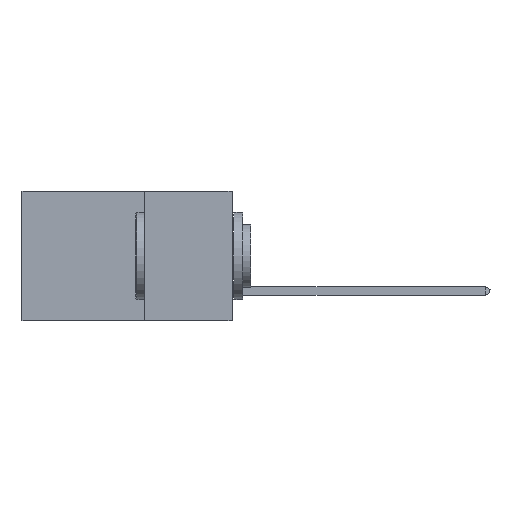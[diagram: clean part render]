
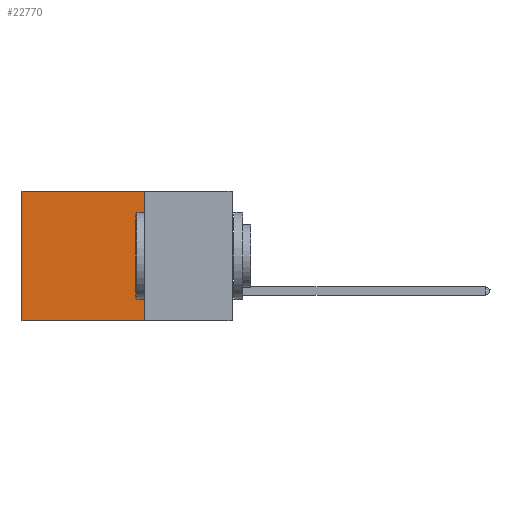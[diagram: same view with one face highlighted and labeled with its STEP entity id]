
A CAD part, left-side view. The second image highlights one B-rep face of the part: STEP entity #22770.
In plain terms, the highlighted planar face has unit normal (-1, 0, 0).
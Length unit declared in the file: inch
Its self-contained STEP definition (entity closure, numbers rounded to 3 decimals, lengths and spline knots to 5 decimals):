
#1149 = PLANE ( 'NONE',  #8282 ) ;
#1723 = VECTOR ( 'NONE', #18892, 39.37008 ) ;
#2273 = VERTEX_POINT ( 'NONE', #7910 ) ;
#2519 = VERTEX_POINT ( 'NONE', #12823 ) ;
#2667 = LINE ( 'NONE', #14567, #1723 ) ;
#3457 = DIRECTION ( 'NONE',  ( 0., 0., -1. ) ) ;
#4595 = VERTEX_POINT ( 'NONE', #13557 ) ;
#5178 = DIRECTION ( 'NONE',  ( 1., 0., 0. ) ) ;
#5205 = ORIENTED_EDGE ( 'NONE', *, *, #19442, .F. ) ;
#5664 = EDGE_CURVE ( 'NONE', #4595, #2273, #2667, .T. ) ;
#6029 = DIRECTION ( 'NONE',  ( 0., 1., 0. ) ) ;
#6645 = CARTESIAN_POINT ( 'NONE',  ( 0.2875, 0.25, 0. ) ) ;
#7910 = CARTESIAN_POINT ( 'NONE',  ( 0.2875, 0.6, -0.37 ) ) ;
#8103 = EDGE_LOOP ( 'NONE', ( #13638, #22200, #5205, #21917 ) ) ;
#8282 = AXIS2_PLACEMENT_3D ( 'NONE', #13088, #5178, #24954 ) ;
#10345 = DIRECTION ( 'NONE',  ( 0., 0., -1. ) ) ;
#10541 = LINE ( 'NONE', #13989, #14677 ) ;
#10616 = LINE ( 'NONE', #18579, #12195 ) ;
#11887 = EDGE_CURVE ( 'NONE', #2519, #2273, #10616, .T. ) ;
#12195 = VECTOR ( 'NONE', #10345, 39.37008 ) ;
#12823 = CARTESIAN_POINT ( 'NONE',  ( 0.2875, 0.6, 0. ) ) ;
#13088 = CARTESIAN_POINT ( 'NONE',  ( 0.2875, 0.25, 0. ) ) ;
#13557 = CARTESIAN_POINT ( 'NONE',  ( 0.2875, 0.25, -0.37 ) ) ;
#13638 = ORIENTED_EDGE ( 'NONE', *, *, #11887, .T. ) ;
#13989 = CARTESIAN_POINT ( 'NONE',  ( 0.2875, 0.25, 0. ) ) ;
#14567 = CARTESIAN_POINT ( 'NONE',  ( 0.2875, 0.25, -0.37 ) ) ;
#14677 = VECTOR ( 'NONE', #6029, 39.37008 ) ;
#15118 = FACE_OUTER_BOUND ( 'NONE', #8103, .T. ) ;
#16511 = CARTESIAN_POINT ( 'NONE',  ( 0.2875, 0.25, 0. ) ) ;
#18579 = CARTESIAN_POINT ( 'NONE',  ( 0.2875, 0.6, 0. ) ) ;
#18892 = DIRECTION ( 'NONE',  ( 0., 1., 0. ) ) ;
#19442 = EDGE_CURVE ( 'NONE', #23478, #4595, #22583, .T. ) ;
#20066 = VECTOR ( 'NONE', #3457, 39.37008 ) ;
#21917 = ORIENTED_EDGE ( 'NONE', *, *, #23062, .T. ) ;
#22200 = ORIENTED_EDGE ( 'NONE', *, *, #5664, .F. ) ;
#22583 = LINE ( 'NONE', #6645, #20066 ) ;
#22770 = ADVANCED_FACE ( 'NONE', ( #15118 ), #1149, .F. ) ;
#23062 = EDGE_CURVE ( 'NONE', #23478, #2519, #10541, .T. ) ;
#23478 = VERTEX_POINT ( 'NONE', #16511 ) ;
#24954 = DIRECTION ( 'NONE',  ( 0., 0., -1. ) ) ;
